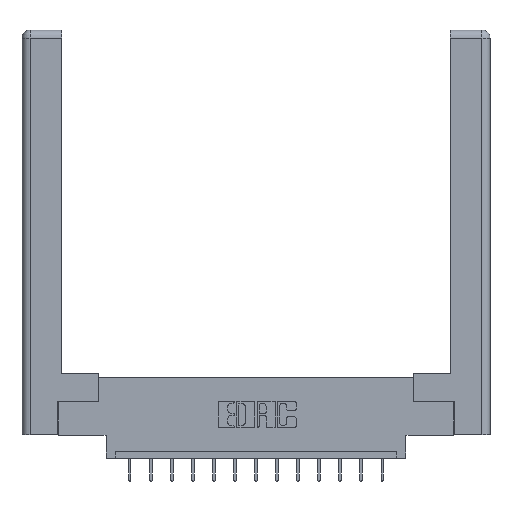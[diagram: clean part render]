
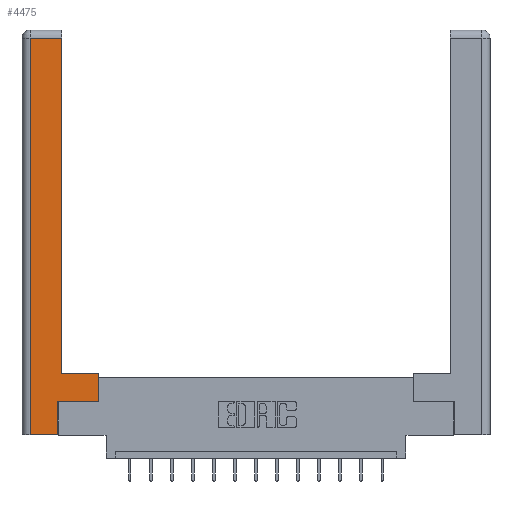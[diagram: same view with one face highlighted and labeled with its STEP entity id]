
A CAD part, top view. The second image highlights one B-rep face of the part: STEP entity #4475.
In plain terms, the highlighted planar face has unit normal (0, 0, 1).
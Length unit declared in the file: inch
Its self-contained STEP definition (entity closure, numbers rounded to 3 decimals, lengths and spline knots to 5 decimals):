
#482 = ORIENTED_EDGE ( 'NONE', *, *, #13793, .T. ) ;
#613 = EDGE_CURVE ( 'NONE', #4968, #625, #15370, .T. ) ;
#625 = VERTEX_POINT ( 'NONE', #12837 ) ;
#702 = ORIENTED_EDGE ( 'NONE', *, *, #15698, .T. ) ;
#856 = ORIENTED_EDGE ( 'NONE', *, *, #10942, .T. ) ;
#1036 = VECTOR ( 'NONE', #8535, 39.37008 ) ;
#1926 = CARTESIAN_POINT ( 'NONE',  ( 0.295, 0.45, 0. ) ) ;
#1996 = DIRECTION ( 'NONE',  ( 1., 0., 0. ) ) ;
#2126 = VECTOR ( 'NONE', #1996, 39.37008 ) ;
#2282 = VERTEX_POINT ( 'NONE', #6841 ) ;
#2468 = VECTOR ( 'NONE', #10263, 39.37008 ) ;
#2509 = CARTESIAN_POINT ( 'NONE',  ( 0., 0., 0. ) ) ;
#2526 = VERTEX_POINT ( 'NONE', #15799 ) ;
#2668 = VECTOR ( 'NONE', #11529, 39.37008 ) ;
#2675 = PLANE ( 'NONE',  #6020 ) ;
#2751 = CARTESIAN_POINT ( 'NONE',  ( 0.0615, 0., 0. ) ) ;
#2843 = CARTESIAN_POINT ( 'NONE',  ( 0.0615, 2.94, 0. ) ) ;
#3065 = VERTEX_POINT ( 'NONE', #1926 ) ;
#3184 = CARTESIAN_POINT ( 'NONE',  ( 0.0615, 0., 0. ) ) ;
#3466 = DIRECTION ( 'NONE',  ( 0., 1., 0. ) ) ;
#3510 = DIRECTION ( 'NONE',  ( 1., 0., 0. ) ) ;
#3521 = CARTESIAN_POINT ( 'NONE',  ( 0.295, 0.45, 0. ) ) ;
#3848 = VERTEX_POINT ( 'NONE', #9874 ) ;
#4206 = CARTESIAN_POINT ( 'NONE',  ( 0.265, 0.245, 0. ) ) ;
#4475 = ADVANCED_FACE ( 'NONE', ( #10545 ), #2675, .F. ) ;
#4495 = LINE ( 'NONE', #14812, #8069 ) ;
#4627 = LINE ( 'NONE', #14106, #2668 ) ;
#4825 = CARTESIAN_POINT ( 'NONE',  ( 0.565, 0.45, 0. ) ) ;
#4968 = VERTEX_POINT ( 'NONE', #9357 ) ;
#6020 = AXIS2_PLACEMENT_3D ( 'NONE', #2509, #7471, #12552 ) ;
#6422 = EDGE_CURVE ( 'NONE', #12625, #3065, #9333, .T. ) ;
#6552 = VECTOR ( 'NONE', #14149, 39.37008 ) ;
#6740 = DIRECTION ( 'NONE',  ( 0., 1., 0. ) ) ;
#6841 = CARTESIAN_POINT ( 'NONE',  ( 0.265, 0., 0. ) ) ;
#7471 = DIRECTION ( 'NONE',  ( 0., 0., -1. ) ) ;
#7614 = VECTOR ( 'NONE', #6740, 39.37008 ) ;
#8069 = VECTOR ( 'NONE', #3510, 39.37008 ) ;
#8535 = DIRECTION ( 'NONE',  ( -1., 0., 0. ) ) ;
#9313 = EDGE_CURVE ( 'NONE', #14205, #2282, #4495, .T. ) ;
#9333 = LINE ( 'NONE', #3521, #1036 ) ;
#9357 = CARTESIAN_POINT ( 'NONE',  ( 0.295, 2.94, 0. ) ) ;
#9445 = ORIENTED_EDGE ( 'NONE', *, *, #9313, .T. ) ;
#9874 = CARTESIAN_POINT ( 'NONE',  ( 0.265, 0.245, 0. ) ) ;
#9974 = ORIENTED_EDGE ( 'NONE', *, *, #10872, .T. ) ;
#10263 = DIRECTION ( 'NONE',  ( 0., -1., 0. ) ) ;
#10311 = CARTESIAN_POINT ( 'NONE',  ( 0.565, 0.45, 0. ) ) ;
#10545 = FACE_OUTER_BOUND ( 'NONE', #12021, .T. ) ;
#10872 = EDGE_CURVE ( 'NONE', #2282, #3848, #10932, .T. ) ;
#10932 = LINE ( 'NONE', #4206, #7614 ) ;
#10942 = EDGE_CURVE ( 'NONE', #625, #14205, #14833, .T. ) ;
#11095 = LINE ( 'NONE', #4825, #14048 ) ;
#11191 = EDGE_CURVE ( 'NONE', #3065, #4968, #4627, .T. ) ;
#11337 = ORIENTED_EDGE ( 'NONE', *, *, #6422, .T. ) ;
#11529 = DIRECTION ( 'NONE',  ( 0., 1., 0. ) ) ;
#12021 = EDGE_LOOP ( 'NONE', ( #15072, #13809, #856, #9445, #9974, #482, #702, #11337 ) ) ;
#12552 = DIRECTION ( 'NONE',  ( -1., 0., 0. ) ) ;
#12625 = VERTEX_POINT ( 'NONE', #10311 ) ;
#12837 = CARTESIAN_POINT ( 'NONE',  ( 0.0615, 2.94, 0. ) ) ;
#13793 = EDGE_CURVE ( 'NONE', #3848, #2526, #14884, .T. ) ;
#13809 = ORIENTED_EDGE ( 'NONE', *, *, #613, .T. ) ;
#14048 = VECTOR ( 'NONE', #3466, 39.37008 ) ;
#14106 = CARTESIAN_POINT ( 'NONE',  ( 0.295, 3., 0. ) ) ;
#14149 = DIRECTION ( 'NONE',  ( -1., 0., 0. ) ) ;
#14205 = VERTEX_POINT ( 'NONE', #3184 ) ;
#14254 = CARTESIAN_POINT ( 'NONE',  ( 0.565, 0.245, 0. ) ) ;
#14812 = CARTESIAN_POINT ( 'NONE',  ( 0.265, 0., 0. ) ) ;
#14833 = LINE ( 'NONE', #2751, #2468 ) ;
#14884 = LINE ( 'NONE', #14254, #2126 ) ;
#15072 = ORIENTED_EDGE ( 'NONE', *, *, #11191, .T. ) ;
#15370 = LINE ( 'NONE', #2843, #6552 ) ;
#15698 = EDGE_CURVE ( 'NONE', #2526, #12625, #11095, .T. ) ;
#15799 = CARTESIAN_POINT ( 'NONE',  ( 0.565, 0.245, 0. ) ) ;
